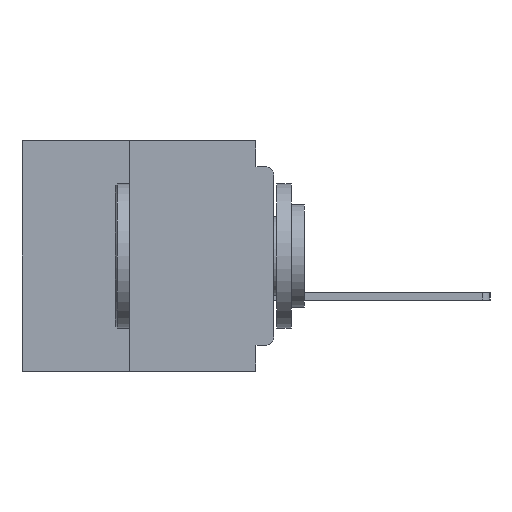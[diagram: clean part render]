
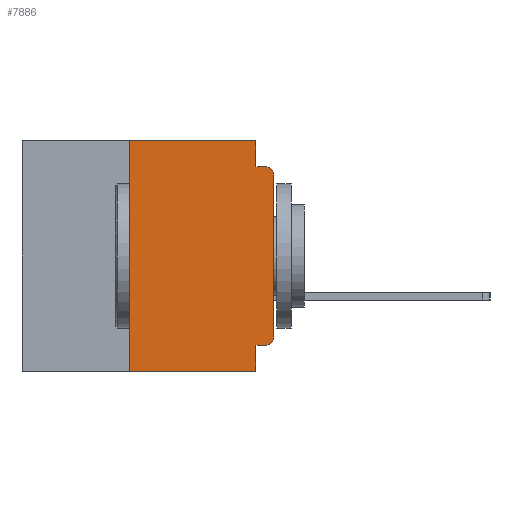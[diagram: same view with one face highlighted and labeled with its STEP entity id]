
A CAD part, left-side view. The second image highlights one B-rep face of the part: STEP entity #7886.
In plain terms, the highlighted planar face has unit normal (-1, 0, 0).
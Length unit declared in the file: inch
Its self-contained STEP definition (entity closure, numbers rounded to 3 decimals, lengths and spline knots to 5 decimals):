
#1 = ORIENTED_EDGE ( 'NONE', *, *, #1866, .T. ) ;
#398 = ORIENTED_EDGE ( 'NONE', *, *, #10266, .F. ) ;
#440 = VECTOR ( 'NONE', #32352, 39.37008 ) ;
#500 = VERTEX_POINT ( 'NONE', #42806 ) ;
#560 = AXIS2_PLACEMENT_3D ( 'NONE', #31393, #31378, #28406 ) ;
#654 = EDGE_CURVE ( 'NONE', #500, #11477, #40330, .T. ) ;
#691 = VECTOR ( 'NONE', #16270, 39.37008 ) ;
#729 = ORIENTED_EDGE ( 'NONE', *, *, #654, .F. ) ;
#1866 = EDGE_CURVE ( 'NONE', #12544, #3993, #45766, .T. ) ;
#1923 = LINE ( 'NONE', #37352, #21039 ) ;
#2347 = FACE_OUTER_BOUND ( 'NONE', #5836, .T. ) ;
#2794 = ORIENTED_EDGE ( 'NONE', *, *, #40288, .F. ) ;
#3993 = VERTEX_POINT ( 'NONE', #16875 ) ;
#4130 = DIRECTION ( 'NONE',  ( 0., 0., -1. ) ) ;
#5676 = CARTESIAN_POINT ( 'NONE',  ( 0., 0.015, -0.355 ) ) ;
#5717 = EDGE_CURVE ( 'NONE', #11477, #22988, #1923, .T. ) ;
#5836 = EDGE_LOOP ( 'NONE', ( #17931, #1, #2794, #398, #43133, #729, #42810, #30553, #24518, #20951 ) ) ;
#5946 = LINE ( 'NONE', #20967, #33419 ) ;
#5963 = VERTEX_POINT ( 'NONE', #31709 ) ;
#6689 = CARTESIAN_POINT ( 'NONE',  ( 0., 0., 0. ) ) ;
#7886 = ADVANCED_FACE ( 'NONE', ( #2347 ), #43193, .F. ) ;
#9137 = CARTESIAN_POINT ( 'NONE',  ( 0., 0., -0.045 ) ) ;
#9302 = CARTESIAN_POINT ( 'NONE',  ( 0., 0.031, -0.355 ) ) ;
#10016 = CARTESIAN_POINT ( 'NONE',  ( 0., 0.031, 0. ) ) ;
#10141 = DIRECTION ( 'NONE',  ( 0., -1., 0. ) ) ;
#10266 = EDGE_CURVE ( 'NONE', #22988, #16332, #26794, .T. ) ;
#11413 = AXIS2_PLACEMENT_3D ( 'NONE', #36429, #15032, #40031 ) ;
#11477 = VERTEX_POINT ( 'NONE', #18197 ) ;
#11791 = DIRECTION ( 'NONE',  ( 0., 0., 1. ) ) ;
#12544 = VERTEX_POINT ( 'NONE', #13994 ) ;
#12988 = EDGE_CURVE ( 'NONE', #45557, #12544, #33528, .T. ) ;
#13994 = CARTESIAN_POINT ( 'NONE',  ( 0., 0., -0.06 ) ) ;
#14729 = CARTESIAN_POINT ( 'NONE',  ( 0., 0.437, 0. ) ) ;
#15032 = DIRECTION ( 'NONE',  ( -1., 0., 0. ) ) ;
#15192 = VECTOR ( 'NONE', #4130, 39.37008 ) ;
#16270 = DIRECTION ( 'NONE',  ( 0., 1., 0. ) ) ;
#16306 = EDGE_CURVE ( 'NONE', #19952, #40306, #28170, .T. ) ;
#16332 = VERTEX_POINT ( 'NONE', #23627 ) ;
#16875 = CARTESIAN_POINT ( 'NONE',  ( 0., 0.015, -0.045 ) ) ;
#17056 = CARTESIAN_POINT ( 'NONE',  ( 0., 0.25, -0.4 ) ) ;
#17931 = ORIENTED_EDGE ( 'NONE', *, *, #12988, .T. ) ;
#18197 = CARTESIAN_POINT ( 'NONE',  ( 0., 0.25, 0. ) ) ;
#18343 = DIRECTION ( 'NONE',  ( 0., 0., -1. ) ) ;
#19952 = VERTEX_POINT ( 'NONE', #5676 ) ;
#20951 = ORIENTED_EDGE ( 'NONE', *, *, #43575, .T. ) ;
#20967 = CARTESIAN_POINT ( 'NONE',  ( 0., 0.437, -0.4 ) ) ;
#21039 = VECTOR ( 'NONE', #37499, 39.37008 ) ;
#21820 = VECTOR ( 'NONE', #11791, 39.37008 ) ;
#22988 = VERTEX_POINT ( 'NONE', #10016 ) ;
#23058 = LINE ( 'NONE', #9137, #31417 ) ;
#23627 = CARTESIAN_POINT ( 'NONE',  ( 0., 0.031, -0.045 ) ) ;
#24518 = ORIENTED_EDGE ( 'NONE', *, *, #16306, .F. ) ;
#26794 = LINE ( 'NONE', #28767, #440 ) ;
#27965 = CIRCLE ( 'NONE', #11413, 0.015 ) ;
#28170 = LINE ( 'NONE', #44847, #691 ) ;
#28286 = CARTESIAN_POINT ( 'NONE',  ( 0., 0.031, -0.4 ) ) ;
#28371 = AXIS2_PLACEMENT_3D ( 'NONE', #14729, #39751, #18343 ) ;
#28406 = DIRECTION ( 'NONE',  ( 0., 0., -1. ) ) ;
#28767 = CARTESIAN_POINT ( 'NONE',  ( 0., 0.031, 0. ) ) ;
#29668 = DIRECTION ( 'NONE',  ( 0., 0., 1. ) ) ;
#30553 = ORIENTED_EDGE ( 'NONE', *, *, #42361, .F. ) ;
#30806 = VECTOR ( 'NONE', #29668, 39.37008 ) ;
#31378 = DIRECTION ( 'NONE',  ( -1., 0., 0. ) ) ;
#31393 = CARTESIAN_POINT ( 'NONE',  ( 0., 0.015, -0.06 ) ) ;
#31417 = VECTOR ( 'NONE', #34171, 39.37008 ) ;
#31709 = CARTESIAN_POINT ( 'NONE',  ( 0., 0.031, -0.4 ) ) ;
#32352 = DIRECTION ( 'NONE',  ( 0., 0., -1. ) ) ;
#33419 = VECTOR ( 'NONE', #10141, 39.37008 ) ;
#33528 = LINE ( 'NONE', #6689, #21820 ) ;
#34171 = DIRECTION ( 'NONE',  ( 0., -1., 0. ) ) ;
#34196 = LINE ( 'NONE', #28286, #15192 ) ;
#36429 = CARTESIAN_POINT ( 'NONE',  ( 0., 0.015, -0.34 ) ) ;
#36656 = CARTESIAN_POINT ( 'NONE',  ( 0., 0., -0.34 ) ) ;
#37352 = CARTESIAN_POINT ( 'NONE',  ( 0., 0.437, 0. ) ) ;
#37499 = DIRECTION ( 'NONE',  ( 0., -1., 0. ) ) ;
#39751 = DIRECTION ( 'NONE',  ( 1., 0., 0. ) ) ;
#40031 = DIRECTION ( 'NONE',  ( 0., 0., -1. ) ) ;
#40288 = EDGE_CURVE ( 'NONE', #16332, #3993, #23058, .T. ) ;
#40306 = VERTEX_POINT ( 'NONE', #9302 ) ;
#40330 = LINE ( 'NONE', #17056, #30806 ) ;
#42361 = EDGE_CURVE ( 'NONE', #40306, #5963, #34196, .T. ) ;
#42806 = CARTESIAN_POINT ( 'NONE',  ( 0., 0.25, -0.4 ) ) ;
#42810 = ORIENTED_EDGE ( 'NONE', *, *, #44710, .T. ) ;
#43133 = ORIENTED_EDGE ( 'NONE', *, *, #5717, .F. ) ;
#43193 = PLANE ( 'NONE',  #28371 ) ;
#43575 = EDGE_CURVE ( 'NONE', #19952, #45557, #27965, .T. ) ;
#44710 = EDGE_CURVE ( 'NONE', #500, #5963, #5946, .T. ) ;
#44847 = CARTESIAN_POINT ( 'NONE',  ( 0., 0., -0.355 ) ) ;
#45557 = VERTEX_POINT ( 'NONE', #36656 ) ;
#45766 = CIRCLE ( 'NONE', #560, 0.015 ) ;
